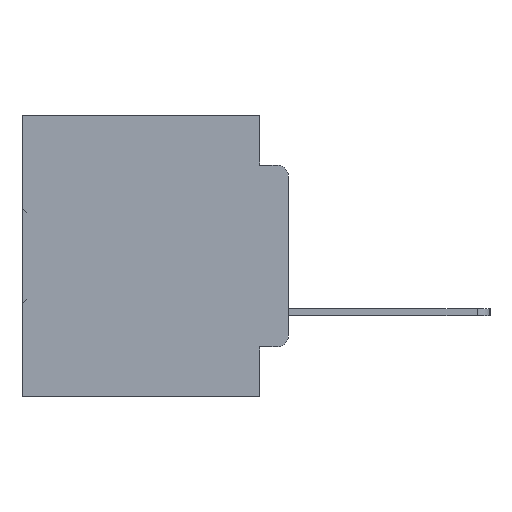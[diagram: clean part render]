
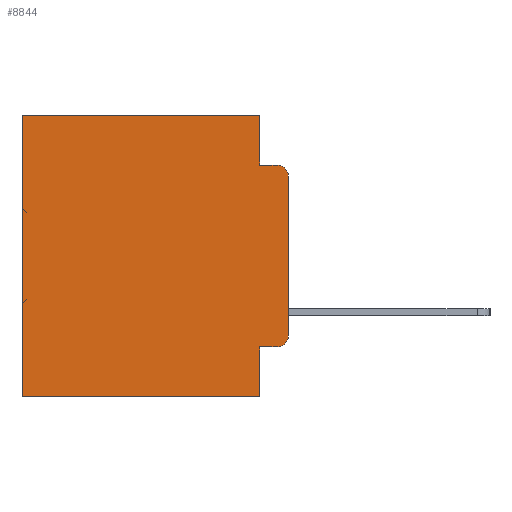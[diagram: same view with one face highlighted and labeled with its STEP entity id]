
A CAD part, left-side view. The second image highlights one B-rep face of the part: STEP entity #8844.
In plain terms, the highlighted planar face has unit normal (-1, 0, 0).
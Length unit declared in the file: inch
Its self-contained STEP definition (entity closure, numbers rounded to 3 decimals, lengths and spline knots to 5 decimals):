
#1033 = DIRECTION ( 'NONE',  ( -1., 0., 0. ) ) ;
#1382 = EDGE_CURVE ( 'NONE', #23112, #36359, #12226, .T. ) ;
#1430 = CARTESIAN_POINT ( 'NONE',  ( 0.298, 0.02, -0.0885 ) ) ;
#2215 = ORIENTED_EDGE ( 'NONE', *, *, #7583, .T. ) ;
#2890 = VECTOR ( 'NONE', #27904, 39.37008 ) ;
#3351 = LINE ( 'NONE', #6349, #24357 ) ;
#3421 = VERTEX_POINT ( 'NONE', #19403 ) ;
#4351 = AXIS2_PLACEMENT_3D ( 'NONE', #18856, #21804, #4650 ) ;
#4650 = DIRECTION ( 'NONE',  ( 0., 0., -1. ) ) ;
#5148 = CARTESIAN_POINT ( 'NONE',  ( 0.298, 0., 0. ) ) ;
#5972 = VERTEX_POINT ( 'NONE', #32932 ) ;
#6164 = CARTESIAN_POINT ( 'NONE',  ( 0.298, 0.051, -0.0885 ) ) ;
#6349 = CARTESIAN_POINT ( 'NONE',  ( 0.298, 0., 0. ) ) ;
#7388 = EDGE_CURVE ( 'NONE', #5972, #7846, #3351, .T. ) ;
#7558 = DIRECTION ( 'NONE',  ( 0., 1., 0. ) ) ;
#7583 = EDGE_CURVE ( 'NONE', #33255, #24987, #10462, .T. ) ;
#7682 = ORIENTED_EDGE ( 'NONE', *, *, #20998, .T. ) ;
#7846 = VERTEX_POINT ( 'NONE', #13246 ) ;
#7902 = LINE ( 'NONE', #6164, #22233 ) ;
#8316 = ORIENTED_EDGE ( 'NONE', *, *, #28628, .F. ) ;
#8844 = ADVANCED_FACE ( 'NONE', ( #26428 ), #35933, .F. ) ;
#8994 = VECTOR ( 'NONE', #36691, 39.37008 ) ;
#10065 = ORIENTED_EDGE ( 'NONE', *, *, #22925, .F. ) ;
#10462 = LINE ( 'NONE', #15640, #2890 ) ;
#11334 = VECTOR ( 'NONE', #19771, 39.37008 ) ;
#11355 = CIRCLE ( 'NONE', #24510, 0.02 ) ;
#11360 = ORIENTED_EDGE ( 'NONE', *, *, #11388, .F. ) ;
#11388 = EDGE_CURVE ( 'NONE', #33255, #23112, #12233, .T. ) ;
#11739 = VERTEX_POINT ( 'NONE', #1430 ) ;
#12226 = LINE ( 'NONE', #15713, #33174 ) ;
#12233 = LINE ( 'NONE', #25529, #11334 ) ;
#12994 = CARTESIAN_POINT ( 'NONE',  ( 0.298, 0.02, -0.3915 ) ) ;
#13246 = CARTESIAN_POINT ( 'NONE',  ( 0.298, 0.473, 0. ) ) ;
#15491 = ORIENTED_EDGE ( 'NONE', *, *, #36928, .T. ) ;
#15640 = CARTESIAN_POINT ( 'NONE',  ( 0.298, 0.051, -0.4115 ) ) ;
#15713 = CARTESIAN_POINT ( 'NONE',  ( 0.298, 0., -0.5 ) ) ;
#15837 = EDGE_LOOP ( 'NONE', ( #35666, #30317, #8316, #10065, #31883, #7682, #30341, #11360, #2215, #15491 ) ) ;
#15857 = DIRECTION ( 'NONE',  ( 0., 0., -1. ) ) ;
#16905 = DIRECTION ( 'NONE',  ( 0., 0., -1. ) ) ;
#17618 = DIRECTION ( 'NONE',  ( 0., -1., 0. ) ) ;
#18089 = CARTESIAN_POINT ( 'NONE',  ( 0.298, 0.02, -0.1085 ) ) ;
#18128 = VERTEX_POINT ( 'NONE', #30384 ) ;
#18856 = CARTESIAN_POINT ( 'NONE',  ( 0.298, 0., 0. ) ) ;
#18869 = CARTESIAN_POINT ( 'NONE',  ( 0.298, 0.051, -0.4115 ) ) ;
#19403 = CARTESIAN_POINT ( 'NONE',  ( 0.298, 0., -0.1085 ) ) ;
#19479 = DIRECTION ( 'NONE',  ( 0., 0., -1. ) ) ;
#19771 = DIRECTION ( 'NONE',  ( 0., 0., -1. ) ) ;
#20998 = EDGE_CURVE ( 'NONE', #7846, #36359, #30722, .T. ) ;
#21013 = DIRECTION ( 'NONE',  ( 0., 0., -1. ) ) ;
#21504 = VECTOR ( 'NONE', #19479, 39.37008 ) ;
#21804 = DIRECTION ( 'NONE',  ( 1., 0., 0. ) ) ;
#22233 = VECTOR ( 'NONE', #17618, 39.37008 ) ;
#22925 = EDGE_CURVE ( 'NONE', #5972, #18128, #23335, .T. ) ;
#23112 = VERTEX_POINT ( 'NONE', #29010 ) ;
#23192 = VECTOR ( 'NONE', #16905, 39.37008 ) ;
#23335 = LINE ( 'NONE', #33818, #8994 ) ;
#23381 = EDGE_CURVE ( 'NONE', #3421, #26222, #29060, .T. ) ;
#24357 = VECTOR ( 'NONE', #31801, 39.37008 ) ;
#24510 = AXIS2_PLACEMENT_3D ( 'NONE', #12994, #32941, #15857 ) ;
#24987 = VERTEX_POINT ( 'NONE', #35558 ) ;
#25529 = CARTESIAN_POINT ( 'NONE',  ( 0.298, 0.051, 0. ) ) ;
#26222 = VERTEX_POINT ( 'NONE', #28784 ) ;
#26428 = FACE_OUTER_BOUND ( 'NONE', #15837, .T. ) ;
#27322 = CARTESIAN_POINT ( 'NONE',  ( 0.298, 0.473, -0.5 ) ) ;
#27904 = DIRECTION ( 'NONE',  ( 0., -1., 0. ) ) ;
#28295 = CARTESIAN_POINT ( 'NONE',  ( 0.298, 0.473, 0. ) ) ;
#28628 = EDGE_CURVE ( 'NONE', #18128, #11739, #7902, .T. ) ;
#28784 = CARTESIAN_POINT ( 'NONE',  ( 0.298, 0., -0.3915 ) ) ;
#29010 = CARTESIAN_POINT ( 'NONE',  ( 0.298, 0.051, -0.5 ) ) ;
#29060 = LINE ( 'NONE', #5148, #21504 ) ;
#30317 = ORIENTED_EDGE ( 'NONE', *, *, #34321, .T. ) ;
#30341 = ORIENTED_EDGE ( 'NONE', *, *, #1382, .F. ) ;
#30384 = CARTESIAN_POINT ( 'NONE',  ( 0.298, 0.051, -0.0885 ) ) ;
#30722 = LINE ( 'NONE', #28295, #23192 ) ;
#30872 = AXIS2_PLACEMENT_3D ( 'NONE', #18089, #1033, #21013 ) ;
#31657 = CIRCLE ( 'NONE', #30872, 0.02 ) ;
#31801 = DIRECTION ( 'NONE',  ( 0., 1., 0. ) ) ;
#31883 = ORIENTED_EDGE ( 'NONE', *, *, #7388, .T. ) ;
#32932 = CARTESIAN_POINT ( 'NONE',  ( 0.298, 0.051, 0. ) ) ;
#32941 = DIRECTION ( 'NONE',  ( -1., 0., 0. ) ) ;
#33174 = VECTOR ( 'NONE', #7558, 39.37008 ) ;
#33255 = VERTEX_POINT ( 'NONE', #18869 ) ;
#33818 = CARTESIAN_POINT ( 'NONE',  ( 0.298, 0.051, 0. ) ) ;
#34321 = EDGE_CURVE ( 'NONE', #3421, #11739, #31657, .T. ) ;
#35558 = CARTESIAN_POINT ( 'NONE',  ( 0.298, 0.02, -0.4115 ) ) ;
#35666 = ORIENTED_EDGE ( 'NONE', *, *, #23381, .F. ) ;
#35933 = PLANE ( 'NONE',  #4351 ) ;
#36359 = VERTEX_POINT ( 'NONE', #27322 ) ;
#36691 = DIRECTION ( 'NONE',  ( 0., 0., -1. ) ) ;
#36928 = EDGE_CURVE ( 'NONE', #24987, #26222, #11355, .T. ) ;
